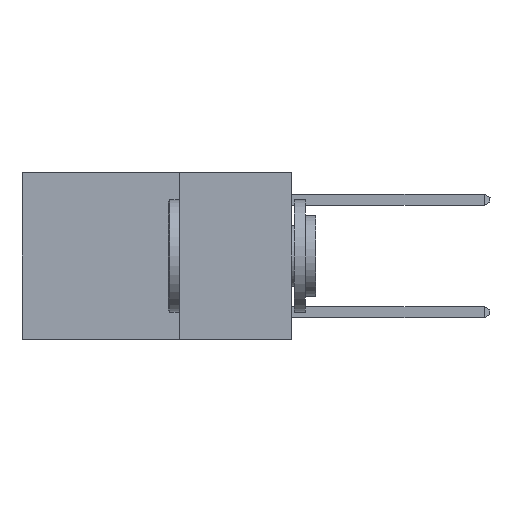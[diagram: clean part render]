
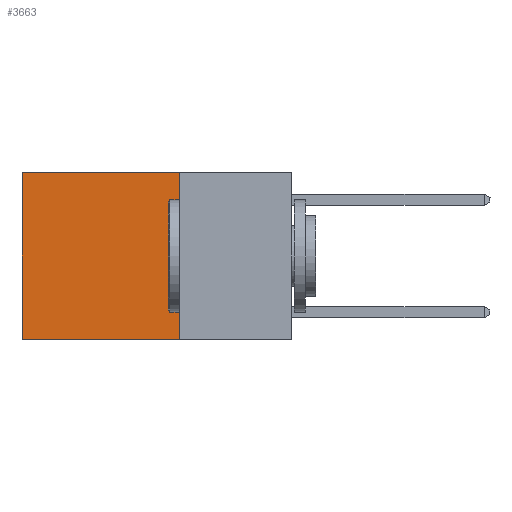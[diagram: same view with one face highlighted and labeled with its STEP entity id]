
A CAD part, left-side view. The second image highlights one B-rep face of the part: STEP entity #3663.
In plain terms, the highlighted planar face has unit normal (-1, 0, 0).
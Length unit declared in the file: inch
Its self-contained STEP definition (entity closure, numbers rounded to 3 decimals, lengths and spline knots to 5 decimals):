
#489 = LINE ( 'NONE', #17475, #7378 ) ;
#1107 = VECTOR ( 'NONE', #10837, 39.37008 ) ;
#2320 = DIRECTION ( 'NONE',  ( 0., 1., 0. ) ) ;
#3650 = ORIENTED_EDGE ( 'NONE', *, *, #22439, .T. ) ;
#3663 = ADVANCED_FACE ( 'NONE', ( #9882 ), #14849, .F. ) ;
#4233 = VERTEX_POINT ( 'NONE', #19620 ) ;
#4708 = CARTESIAN_POINT ( 'NONE',  ( 0.2625, 0.25, -0.37 ) ) ;
#5417 = EDGE_CURVE ( 'NONE', #28870, #19037, #21570, .T. ) ;
#5624 = DIRECTION ( 'NONE',  ( 0., 1., 0. ) ) ;
#7378 = VECTOR ( 'NONE', #5624, 39.37008 ) ;
#7807 = DIRECTION ( 'NONE',  ( 1., 0., 0. ) ) ;
#7962 = CARTESIAN_POINT ( 'NONE',  ( 0.2625, 0.25, 0. ) ) ;
#9071 = VECTOR ( 'NONE', #2320, 39.37008 ) ;
#9882 = FACE_OUTER_BOUND ( 'NONE', #16688, .T. ) ;
#10837 = DIRECTION ( 'NONE',  ( 0., 0., -1. ) ) ;
#14849 = PLANE ( 'NONE',  #31325 ) ;
#16688 = EDGE_LOOP ( 'NONE', ( #3650, #20146, #30086, #18562 ) ) ;
#16918 = DIRECTION ( 'NONE',  ( 0., 0., -1. ) ) ;
#17228 = CARTESIAN_POINT ( 'NONE',  ( 0.2625, 0.6, 0. ) ) ;
#17475 = CARTESIAN_POINT ( 'NONE',  ( 0.2625, 0.25, -0.37 ) ) ;
#18562 = ORIENTED_EDGE ( 'NONE', *, *, #5417, .T. ) ;
#19037 = VERTEX_POINT ( 'NONE', #21916 ) ;
#19227 = EDGE_CURVE ( 'NONE', #28870, #25470, #23039, .T. ) ;
#19620 = CARTESIAN_POINT ( 'NONE',  ( 0.2625, 0.6, -0.37 ) ) ;
#20146 = ORIENTED_EDGE ( 'NONE', *, *, #24678, .F. ) ;
#21570 = LINE ( 'NONE', #28799, #9071 ) ;
#21916 = CARTESIAN_POINT ( 'NONE',  ( 0.2625, 0.6, 0. ) ) ;
#22439 = EDGE_CURVE ( 'NONE', #19037, #4233, #24467, .T. ) ;
#23039 = LINE ( 'NONE', #7962, #1107 ) ;
#24296 = VECTOR ( 'NONE', #16918, 39.37008 ) ;
#24467 = LINE ( 'NONE', #17228, #24296 ) ;
#24678 = EDGE_CURVE ( 'NONE', #25470, #4233, #489, .T. ) ;
#25136 = CARTESIAN_POINT ( 'NONE',  ( 0.2625, 0.25, 0. ) ) ;
#25470 = VERTEX_POINT ( 'NONE', #4708 ) ;
#28799 = CARTESIAN_POINT ( 'NONE',  ( 0.2625, 0.25, 0. ) ) ;
#28870 = VERTEX_POINT ( 'NONE', #30985 ) ;
#30086 = ORIENTED_EDGE ( 'NONE', *, *, #19227, .F. ) ;
#30095 = DIRECTION ( 'NONE',  ( 0., 0., -1. ) ) ;
#30985 = CARTESIAN_POINT ( 'NONE',  ( 0.2625, 0.25, 0. ) ) ;
#31325 = AXIS2_PLACEMENT_3D ( 'NONE', #25136, #7807, #30095 ) ;
